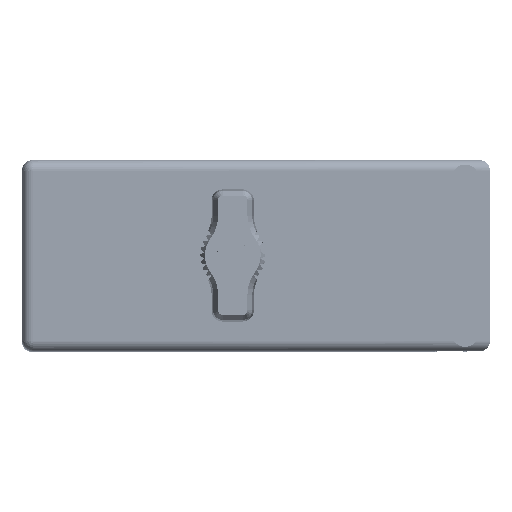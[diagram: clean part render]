
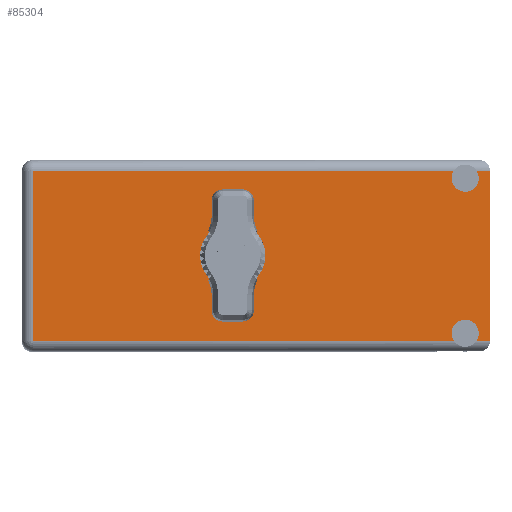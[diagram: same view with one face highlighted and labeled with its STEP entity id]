
A CAD part, top view. The second image highlights one B-rep face of the part: STEP entity #85304.
In plain terms, the highlighted face is planar.
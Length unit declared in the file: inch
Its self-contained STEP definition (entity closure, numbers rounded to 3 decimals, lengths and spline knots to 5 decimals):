
#1728 = CARTESIAN_POINT ( 'NONE',  ( 2.858, 1.775, -1.117 ) ) ;
#4011 = EDGE_CURVE ( 'NONE', #18510, #82737, #88453, .T. ) ;
#5802 = DIRECTION ( 'NONE',  ( 0., 1., 0. ) ) ;
#6603 = ORIENTED_EDGE ( 'NONE', *, *, #39341, .F. ) ;
#6604 = CARTESIAN_POINT ( 'NONE',  ( 2.858, 1.775, -1.117 ) ) ;
#7064 = ORIENTED_EDGE ( 'NONE', *, *, #70314, .F. ) ;
#7355 = DIRECTION ( 'NONE',  ( 0., 1., 0. ) ) ;
#7519 = AXIS2_PLACEMENT_3D ( 'NONE', #81713, #5802, #39718 ) ;
#8620 = EDGE_LOOP ( 'NONE', ( #38044, #7064 ) ) ;
#9035 = ORIENTED_EDGE ( 'NONE', *, *, #83225, .T. ) ;
#9095 = CARTESIAN_POINT ( 'NONE',  ( 2.93181, 1.775, -0.07 ) ) ;
#9781 = ORIENTED_EDGE ( 'NONE', *, *, #32410, .F. ) ;
#10633 = VERTEX_POINT ( 'NONE', #69059 ) ;
#11942 = CARTESIAN_POINT ( 'NONE',  ( 0., 1.775, -1.234 ) ) ;
#13526 = VERTEX_POINT ( 'NONE', #59234 ) ;
#13861 = EDGE_CURVE ( 'NONE', #64473, #13526, #52236, .T. ) ;
#14472 = ORIENTED_EDGE ( 'NONE', *, *, #51808, .T. ) ;
#14758 = CIRCLE ( 'NONE', #7519, 0.0875 ) ;
#15296 = CARTESIAN_POINT ( 'NONE',  ( 3.018, 1.775, -0.07 ) ) ;
#16346 = VECTOR ( 'NONE', #55108, 39.37008 ) ;
#17838 = FACE_BOUND ( 'NONE', #8620, .T. ) ;
#18010 = DIRECTION ( 'NONE',  ( 0., 1., 0. ) ) ;
#18510 = VERTEX_POINT ( 'NONE', #62242 ) ;
#20420 = DIRECTION ( 'NONE',  ( 0., 0., 1. ) ) ;
#23352 = DIRECTION ( 'NONE',  ( 0., 1., 0. ) ) ;
#25011 = VECTOR ( 'NONE', #20420, 39.37008 ) ;
#26522 = CARTESIAN_POINT ( 'NONE',  ( 1.359, 1.775, -0.492 ) ) ;
#27551 = CARTESIAN_POINT ( 'NONE',  ( 0., 1.775, -1.164 ) ) ;
#29231 = CARTESIAN_POINT ( 'NONE',  ( 1.359, 1.775, -0.617 ) ) ;
#31372 = DIRECTION ( 'NONE',  ( -1., 0., 0. ) ) ;
#31815 = LINE ( 'NONE', #39487, #60929 ) ;
#32410 = EDGE_CURVE ( 'NONE', #55180, #85344, #33238, .T. ) ;
#33238 = CIRCLE ( 'NONE', #59038, 0.0875 ) ;
#33519 = CARTESIAN_POINT ( 'NONE',  ( 2.78419, 1.775, -1.164 ) ) ;
#34340 = LINE ( 'NONE', #27551, #16346 ) ;
#34599 = ORIENTED_EDGE ( 'NONE', *, *, #53117, .F. ) ;
#34976 = ORIENTED_EDGE ( 'NONE', *, *, #4011, .F. ) ;
#36551 = DIRECTION ( 'NONE',  ( 1., 0., 0. ) ) ;
#38044 = ORIENTED_EDGE ( 'NONE', *, *, #45801, .F. ) ;
#39341 = EDGE_CURVE ( 'NONE', #85344, #13526, #14758, .T. ) ;
#39487 = CARTESIAN_POINT ( 'NONE',  ( 0., 1.775, -1.164 ) ) ;
#39718 = DIRECTION ( 'NONE',  ( 0., 0., 1. ) ) ;
#40562 = AXIS2_PLACEMENT_3D ( 'NONE', #50318, #7355, #62486 ) ;
#42011 = EDGE_CURVE ( 'NONE', #74093, #64473, #88239, .T. ) ;
#42443 = CARTESIAN_POINT ( 'NONE',  ( 0.07, 1.775, -0.07 ) ) ;
#43772 = AXIS2_PLACEMENT_3D ( 'NONE', #1728, #84420, #70861 ) ;
#44914 = AXIS2_PLACEMENT_3D ( 'NONE', #11942, #80200, #74738 ) ;
#45339 = VECTOR ( 'NONE', #50916, 39.37008 ) ;
#45801 = EDGE_CURVE ( 'NONE', #79645, #82959, #76031, .T. ) ;
#46033 = CARTESIAN_POINT ( 'NONE',  ( 2.858, 1.775, -0.117 ) ) ;
#46730 = PLANE ( 'NONE',  #44914 ) ;
#47286 = AXIS2_PLACEMENT_3D ( 'NONE', #6604, #61290, #82956 ) ;
#50318 = CARTESIAN_POINT ( 'NONE',  ( 1.359, 1.775, -0.617 ) ) ;
#50916 = DIRECTION ( 'NONE',  ( 1., 0., 0. ) ) ;
#51634 = CARTESIAN_POINT ( 'NONE',  ( 3.018, 1.775, -1.164 ) ) ;
#51808 = EDGE_CURVE ( 'NONE', #82596, #74093, #34340, .T. ) ;
#52199 = DIRECTION ( 'NONE',  ( 0., 0., 1. ) ) ;
#52236 = LINE ( 'NONE', #71684, #45339 ) ;
#53117 = EDGE_CURVE ( 'NONE', #70532, #10633, #86999, .T. ) ;
#53311 = CARTESIAN_POINT ( 'NONE',  ( 1.359, 1.775, -0.742 ) ) ;
#54329 = CARTESIAN_POINT ( 'NONE',  ( 0.07, 1.775, -1.234 ) ) ;
#54728 = CARTESIAN_POINT ( 'NONE',  ( 2.93181, 1.775, -1.164 ) ) ;
#55108 = DIRECTION ( 'NONE',  ( -1., 0., 0. ) ) ;
#55180 = VERTEX_POINT ( 'NONE', #9095 ) ;
#56503 = CIRCLE ( 'NONE', #40562, 0.125 ) ;
#58397 = CARTESIAN_POINT ( 'NONE',  ( 0.07, 1.775, -1.164 ) ) ;
#58701 = DIRECTION ( 'NONE',  ( 0., 0., 1. ) ) ;
#59038 = AXIS2_PLACEMENT_3D ( 'NONE', #46033, #18010, #58701 ) ;
#59234 = CARTESIAN_POINT ( 'NONE',  ( 2.78419, 1.775, -0.07 ) ) ;
#60291 = CARTESIAN_POINT ( 'NONE',  ( 2.858, 1.775, -0.2045 ) ) ;
#60929 = VECTOR ( 'NONE', #31372, 39.37008 ) ;
#61259 = ORIENTED_EDGE ( 'NONE', *, *, #73157, .T. ) ;
#61290 = DIRECTION ( 'NONE',  ( 0., 1., 0. ) ) ;
#62242 = CARTESIAN_POINT ( 'NONE',  ( 2.858, 1.775, -1.0295 ) ) ;
#62486 = DIRECTION ( 'NONE',  ( 0., 0., 1. ) ) ;
#63137 = CIRCLE ( 'NONE', #47286, 0.0875 ) ;
#63547 = DIRECTION ( 'NONE',  ( 0., 0., 1. ) ) ;
#64195 = VECTOR ( 'NONE', #52199, 39.37008 ) ;
#64473 = VERTEX_POINT ( 'NONE', #42443 ) ;
#66407 = EDGE_CURVE ( 'NONE', #82596, #18510, #63137, .T. ) ;
#68155 = ORIENTED_EDGE ( 'NONE', *, *, #66407, .F. ) ;
#69059 = CARTESIAN_POINT ( 'NONE',  ( 3.018, 1.775, -0.07 ) ) ;
#69228 = ORIENTED_EDGE ( 'NONE', *, *, #42011, .T. ) ;
#70107 = ORIENTED_EDGE ( 'NONE', *, *, #13861, .T. ) ;
#70314 = EDGE_CURVE ( 'NONE', #82959, #79645, #56503, .T. ) ;
#70532 = VERTEX_POINT ( 'NONE', #51634 ) ;
#70854 = VECTOR ( 'NONE', #36551, 39.37008 ) ;
#70861 = DIRECTION ( 'NONE',  ( 0., 0., 1. ) ) ;
#71684 = CARTESIAN_POINT ( 'NONE',  ( 3.018, 1.775, -0.07 ) ) ;
#73157 = EDGE_CURVE ( 'NONE', #70532, #82737, #31815, .T. ) ;
#74093 = VERTEX_POINT ( 'NONE', #58397 ) ;
#74738 = DIRECTION ( 'NONE',  ( 0., 0., 1. ) ) ;
#76031 = CIRCLE ( 'NONE', #77468, 0.125 ) ;
#77468 = AXIS2_PLACEMENT_3D ( 'NONE', #29231, #23352, #63547 ) ;
#79645 = VERTEX_POINT ( 'NONE', #26522 ) ;
#80200 = DIRECTION ( 'NONE',  ( 0., 1., 0. ) ) ;
#80687 = EDGE_LOOP ( 'NONE', ( #70107, #6603, #9781, #9035, #34599, #61259, #34976, #68155, #14472, #69228 ) ) ;
#81713 = CARTESIAN_POINT ( 'NONE',  ( 2.858, 1.775, -0.117 ) ) ;
#82596 = VERTEX_POINT ( 'NONE', #33519 ) ;
#82737 = VERTEX_POINT ( 'NONE', #54728 ) ;
#82956 = DIRECTION ( 'NONE',  ( 0., 0., 1. ) ) ;
#82959 = VERTEX_POINT ( 'NONE', #53311 ) ;
#83225 = EDGE_CURVE ( 'NONE', #55180, #10633, #85329, .T. ) ;
#84420 = DIRECTION ( 'NONE',  ( 0., 1., 0. ) ) ;
#85304 = ADVANCED_FACE ( 'NONE', ( #17838, #87866 ), #46730, .T. ) ;
#85329 = LINE ( 'NONE', #15296, #70854 ) ;
#85344 = VERTEX_POINT ( 'NONE', #60291 ) ;
#86999 = LINE ( 'NONE', #87442, #64195 ) ;
#87442 = CARTESIAN_POINT ( 'NONE',  ( 3.018, 1.775, 0. ) ) ;
#87866 = FACE_OUTER_BOUND ( 'NONE', #80687, .T. ) ;
#88239 = LINE ( 'NONE', #54329, #25011 ) ;
#88453 = CIRCLE ( 'NONE', #43772, 0.0875 ) ;
